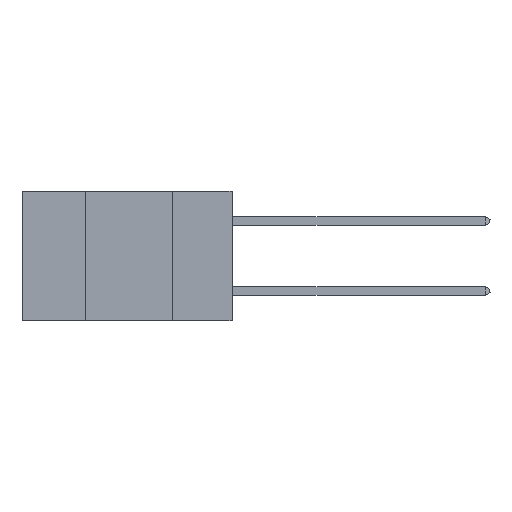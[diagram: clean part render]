
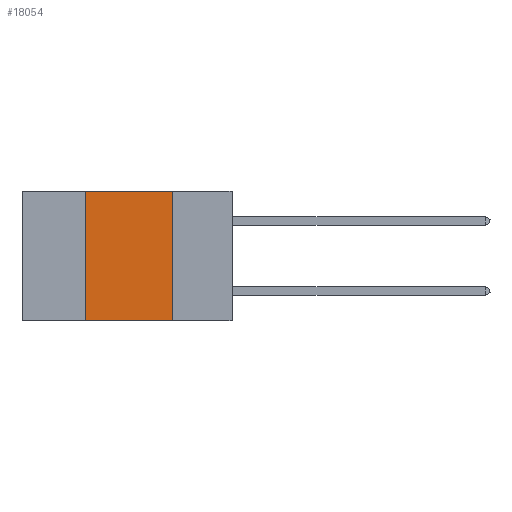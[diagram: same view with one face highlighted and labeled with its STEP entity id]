
A CAD part, left-side view. The second image highlights one B-rep face of the part: STEP entity #18054.
In plain terms, the highlighted planar face has unit normal (-1, 0, 0).
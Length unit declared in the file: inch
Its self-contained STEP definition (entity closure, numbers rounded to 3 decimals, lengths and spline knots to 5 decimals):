
#330 = LINE ( 'NONE', #2184, #29874 ) ;
#769 = CARTESIAN_POINT ( 'NONE',  ( 0., 0.42, 0. ) ) ;
#899 = CARTESIAN_POINT ( 'NONE',  ( 0., 0.17, 0. ) ) ;
#1177 = EDGE_CURVE ( 'NONE', #11497, #26600, #330, .T. ) ;
#2184 = CARTESIAN_POINT ( 'NONE',  ( 0., 0.6, -0.37 ) ) ;
#2940 = VECTOR ( 'NONE', #9192, 39.37008 ) ;
#7082 = CARTESIAN_POINT ( 'NONE',  ( 0., 0.6, 0. ) ) ;
#7322 = PLANE ( 'NONE',  #34999 ) ;
#7374 = LINE ( 'NONE', #26844, #36860 ) ;
#8484 = FACE_OUTER_BOUND ( 'NONE', #33828, .T. ) ;
#9192 = DIRECTION ( 'NONE',  ( 0., 0., -1. ) ) ;
#9281 = DIRECTION ( 'NONE',  ( 0., -1., 0. ) ) ;
#10370 = ORIENTED_EDGE ( 'NONE', *, *, #20785, .F. ) ;
#11497 = VERTEX_POINT ( 'NONE', #23606 ) ;
#12086 = CARTESIAN_POINT ( 'NONE',  ( 0., 0.17, 0. ) ) ;
#12613 = EDGE_CURVE ( 'NONE', #19817, #28377, #7374, .T. ) ;
#18054 = ADVANCED_FACE ( 'NONE', ( #8484 ), #7322, .F. ) ;
#18479 = DIRECTION ( 'NONE',  ( 0., 0., -1. ) ) ;
#19817 = VERTEX_POINT ( 'NONE', #769 ) ;
#19827 = DIRECTION ( 'NONE',  ( 0., -1., 0. ) ) ;
#20348 = EDGE_CURVE ( 'NONE', #11497, #19817, #23999, .T. ) ;
#20785 = EDGE_CURVE ( 'NONE', #28377, #26600, #33771, .T. ) ;
#21439 = ORIENTED_EDGE ( 'NONE', *, *, #1177, .T. ) ;
#23168 = ORIENTED_EDGE ( 'NONE', *, *, #12613, .F. ) ;
#23606 = CARTESIAN_POINT ( 'NONE',  ( 0., 0.42, -0.37 ) ) ;
#23999 = LINE ( 'NONE', #34801, #25773 ) ;
#25773 = VECTOR ( 'NONE', #32914, 39.37008 ) ;
#26600 = VERTEX_POINT ( 'NONE', #27933 ) ;
#26844 = CARTESIAN_POINT ( 'NONE',  ( 0., 0.6, 0. ) ) ;
#27933 = CARTESIAN_POINT ( 'NONE',  ( 0., 0.17, -0.37 ) ) ;
#28377 = VERTEX_POINT ( 'NONE', #899 ) ;
#29874 = VECTOR ( 'NONE', #19827, 39.37008 ) ;
#30325 = ORIENTED_EDGE ( 'NONE', *, *, #20348, .F. ) ;
#32914 = DIRECTION ( 'NONE',  ( 0., 0., 1. ) ) ;
#33771 = LINE ( 'NONE', #12086, #2940 ) ;
#33828 = EDGE_LOOP ( 'NONE', ( #10370, #23168, #30325, #21439 ) ) ;
#34801 = CARTESIAN_POINT ( 'NONE',  ( 0., 0.42, 0. ) ) ;
#34999 = AXIS2_PLACEMENT_3D ( 'NONE', #7082, #35543, #18479 ) ;
#35543 = DIRECTION ( 'NONE',  ( 1., 0., 0. ) ) ;
#36860 = VECTOR ( 'NONE', #9281, 39.37008 ) ;
